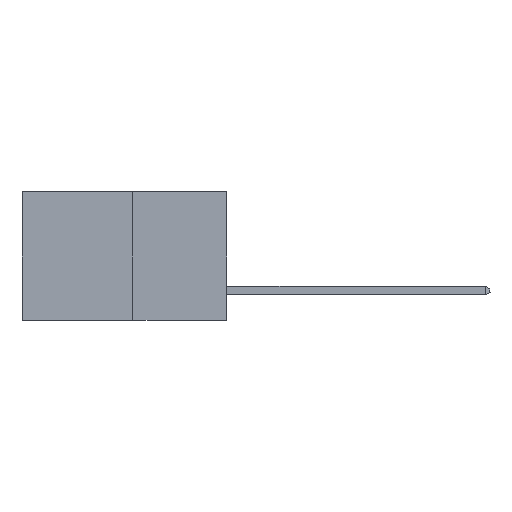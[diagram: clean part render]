
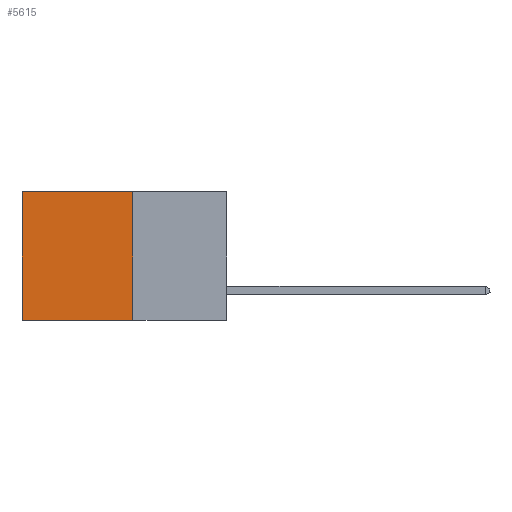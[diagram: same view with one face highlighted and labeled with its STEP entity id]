
A CAD part, left-side view. The second image highlights one B-rep face of the part: STEP entity #5615.
In plain terms, the highlighted planar face has unit normal (-1, 0, 0).
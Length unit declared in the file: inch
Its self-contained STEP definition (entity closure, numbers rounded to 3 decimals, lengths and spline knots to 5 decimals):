
#395 = ORIENTED_EDGE ( 'NONE', *, *, #517, .T. ) ;
#474 = LINE ( 'NONE', #8609, #9324 ) ;
#517 = EDGE_CURVE ( 'NONE', #17959, #2585, #21002, .T. ) ;
#2343 = CARTESIAN_POINT ( 'NONE',  ( 0.277, 0.27, -0.37 ) ) ;
#2535 = VERTEX_POINT ( 'NONE', #22037 ) ;
#2585 = VERTEX_POINT ( 'NONE', #22377 ) ;
#3930 = LINE ( 'NONE', #7359, #12748 ) ;
#4675 = EDGE_CURVE ( 'NONE', #10367, #2535, #15943, .T. ) ;
#4824 = ORIENTED_EDGE ( 'NONE', *, *, #4675, .F. ) ;
#5143 = DIRECTION ( 'NONE',  ( 0., 0., -1. ) ) ;
#5615 = ADVANCED_FACE ( 'NONE', ( #19213 ), #17247, .F. ) ;
#7359 = CARTESIAN_POINT ( 'NONE',  ( 0.277, 0.27, -0.37 ) ) ;
#8609 = CARTESIAN_POINT ( 'NONE',  ( 0.277, 0.59, -0.37 ) ) ;
#9134 = DIRECTION ( 'NONE',  ( 0., 0., -1. ) ) ;
#9324 = VECTOR ( 'NONE', #5143, 39.37008 ) ;
#10367 = VERTEX_POINT ( 'NONE', #2343 ) ;
#11363 = VECTOR ( 'NONE', #20966, 39.37008 ) ;
#11465 = EDGE_CURVE ( 'NONE', #2585, #2535, #474, .T. ) ;
#11673 = EDGE_LOOP ( 'NONE', ( #19718, #4824, #13674, #395 ) ) ;
#11717 = CARTESIAN_POINT ( 'NONE',  ( 0.277, 0.27, 0. ) ) ;
#12748 = VECTOR ( 'NONE', #9134, 39.37008 ) ;
#13674 = ORIENTED_EDGE ( 'NONE', *, *, #14466, .F. ) ;
#14293 = CARTESIAN_POINT ( 'NONE',  ( 0.277, 0.27, -0.37 ) ) ;
#14466 = EDGE_CURVE ( 'NONE', #17959, #10367, #3930, .T. ) ;
#15364 = CARTESIAN_POINT ( 'NONE',  ( 0.277, 0.27, 0. ) ) ;
#15943 = LINE ( 'NONE', #21401, #11363 ) ;
#17080 = DIRECTION ( 'NONE',  ( 0., 0., -1. ) ) ;
#17123 = DIRECTION ( 'NONE',  ( 1., 0., 0. ) ) ;
#17247 = PLANE ( 'NONE',  #21316 ) ;
#17959 = VERTEX_POINT ( 'NONE', #15364 ) ;
#19213 = FACE_OUTER_BOUND ( 'NONE', #11673, .T. ) ;
#19718 = ORIENTED_EDGE ( 'NONE', *, *, #11465, .T. ) ;
#20966 = DIRECTION ( 'NONE',  ( 0., 1., 0. ) ) ;
#21002 = LINE ( 'NONE', #11717, #21535 ) ;
#21316 = AXIS2_PLACEMENT_3D ( 'NONE', #14293, #17123, #17080 ) ;
#21401 = CARTESIAN_POINT ( 'NONE',  ( 0.277, 0.27, -0.37 ) ) ;
#21535 = VECTOR ( 'NONE', #22157, 39.37008 ) ;
#22037 = CARTESIAN_POINT ( 'NONE',  ( 0.277, 0.59, -0.37 ) ) ;
#22157 = DIRECTION ( 'NONE',  ( 0., 1., 0. ) ) ;
#22377 = CARTESIAN_POINT ( 'NONE',  ( 0.277, 0.59, 0. ) ) ;
